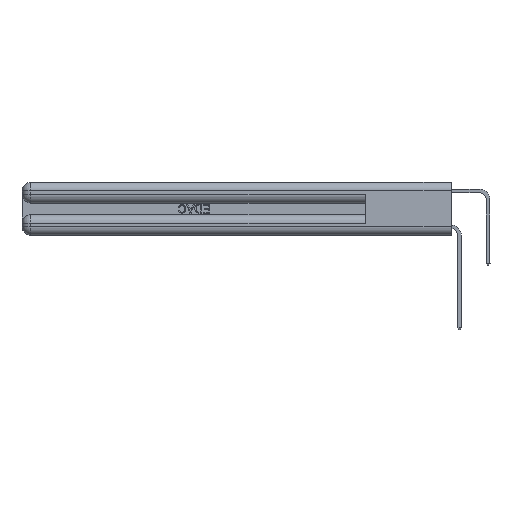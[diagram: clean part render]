
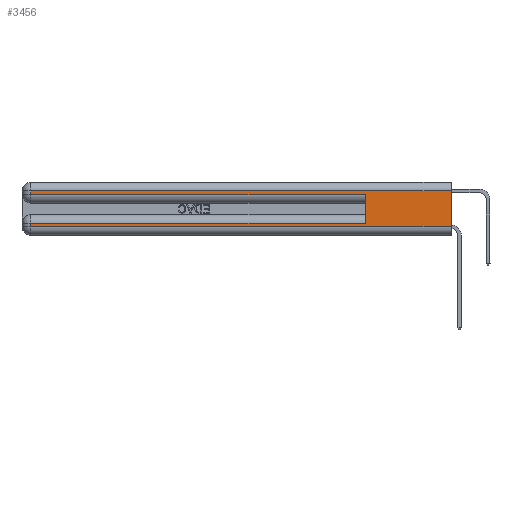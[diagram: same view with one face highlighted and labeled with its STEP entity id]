
A CAD part, left-side view. The second image highlights one B-rep face of the part: STEP entity #3456.
In plain terms, the highlighted planar face has unit normal (-1, 0, 0).
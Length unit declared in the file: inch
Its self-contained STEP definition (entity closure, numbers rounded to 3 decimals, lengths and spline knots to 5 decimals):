
#1261 = ORIENTED_EDGE ( 'NONE', *, *, #28206, .T. ) ;
#2164 = VERTEX_POINT ( 'NONE', #16206 ) ;
#2178 = EDGE_LOOP ( 'NONE', ( #3688, #9739, #6371, #5491, #11661, #1261, #35251, #3676 ) ) ;
#2250 = DIRECTION ( 'NONE',  ( 0., 0., -1. ) ) ;
#2482 = EDGE_CURVE ( 'NONE', #33206, #17365, #23235, .T. ) ;
#2525 = LINE ( 'NONE', #25036, #19591 ) ;
#2604 = FACE_OUTER_BOUND ( 'NONE', #2178, .T. ) ;
#2754 = CARTESIAN_POINT ( 'NONE',  ( 0., 0.6, 0.285 ) ) ;
#3178 = CARTESIAN_POINT ( 'NONE',  ( 0., 2.94, 0.31 ) ) ;
#3456 = ADVANCED_FACE ( 'NONE', ( #2604 ), #27285, .F. ) ;
#3676 = ORIENTED_EDGE ( 'NONE', *, *, #5125, .T. ) ;
#3688 = ORIENTED_EDGE ( 'NONE', *, *, #35032, .F. ) ;
#4379 = DIRECTION ( 'NONE',  ( 0., -1., 0. ) ) ;
#5125 = EDGE_CURVE ( 'NONE', #19645, #2164, #34549, .T. ) ;
#5234 = VECTOR ( 'NONE', #4379, 39.37008 ) ;
#5433 = VERTEX_POINT ( 'NONE', #14145 ) ;
#5491 = ORIENTED_EDGE ( 'NONE', *, *, #6672, .T. ) ;
#5959 = DIRECTION ( 'NONE',  ( 0., 0., -1. ) ) ;
#6371 = ORIENTED_EDGE ( 'NONE', *, *, #25532, .T. ) ;
#6623 = DIRECTION ( 'NONE',  ( 0., 1., 0. ) ) ;
#6672 = EDGE_CURVE ( 'NONE', #34575, #17365, #23557, .T. ) ;
#6862 = CARTESIAN_POINT ( 'NONE',  ( 0., 0., 0.31 ) ) ;
#7670 = VECTOR ( 'NONE', #18965, 39.37008 ) ;
#8605 = VECTOR ( 'NONE', #23261, 39.37008 ) ;
#8687 = LINE ( 'NONE', #27929, #15969 ) ;
#9184 = LINE ( 'NONE', #23133, #9916 ) ;
#9739 = ORIENTED_EDGE ( 'NONE', *, *, #32189, .T. ) ;
#9916 = VECTOR ( 'NONE', #6623, 39.37008 ) ;
#11070 = DIRECTION ( 'NONE',  ( 0., 0., -1. ) ) ;
#11502 = VERTEX_POINT ( 'NONE', #3178 ) ;
#11661 = ORIENTED_EDGE ( 'NONE', *, *, #2482, .F. ) ;
#13624 = VERTEX_POINT ( 'NONE', #6862 ) ;
#14145 = CARTESIAN_POINT ( 'NONE',  ( 0., 2.94, 0.085 ) ) ;
#14431 = EDGE_CURVE ( 'NONE', #5433, #19645, #34548, .T. ) ;
#15689 = CARTESIAN_POINT ( 'NONE',  ( 0., 2.94, 0.06 ) ) ;
#15969 = VECTOR ( 'NONE', #5959, 39.37008 ) ;
#16206 = CARTESIAN_POINT ( 'NONE',  ( 0., 0., 0.06 ) ) ;
#17365 = VERTEX_POINT ( 'NONE', #2754 ) ;
#17774 = CARTESIAN_POINT ( 'NONE',  ( 0., 0.6, 0.145 ) ) ;
#18348 = CARTESIAN_POINT ( 'NONE',  ( 0., 0., 0.06 ) ) ;
#18965 = DIRECTION ( 'NONE',  ( 0., 1., 0. ) ) ;
#19591 = VECTOR ( 'NONE', #11070, 39.37008 ) ;
#19618 = CARTESIAN_POINT ( 'NONE',  ( 0., 2.94, 0.285 ) ) ;
#19645 = VERTEX_POINT ( 'NONE', #15689 ) ;
#20092 = CARTESIAN_POINT ( 'NONE',  ( 0., 0.6, 0.085 ) ) ;
#20697 = CARTESIAN_POINT ( 'NONE',  ( 0., 2.94, 0.37 ) ) ;
#21328 = CARTESIAN_POINT ( 'NONE',  ( 0., 0., 0.31 ) ) ;
#23133 = CARTESIAN_POINT ( 'NONE',  ( 0., 0., 0.085 ) ) ;
#23235 = LINE ( 'NONE', #17774, #31359 ) ;
#23261 = DIRECTION ( 'NONE',  ( 0., 0., -1. ) ) ;
#23380 = CARTESIAN_POINT ( 'NONE',  ( 0., 0., 0.285 ) ) ;
#23557 = LINE ( 'NONE', #23380, #34539 ) ;
#24200 = CARTESIAN_POINT ( 'NONE',  ( 0., 0., 0.37 ) ) ;
#24245 = LINE ( 'NONE', #21328, #7670 ) ;
#25036 = CARTESIAN_POINT ( 'NONE',  ( 0., 0., 0.37 ) ) ;
#25532 = EDGE_CURVE ( 'NONE', #11502, #34575, #8687, .T. ) ;
#27285 = PLANE ( 'NONE',  #29487 ) ;
#27929 = CARTESIAN_POINT ( 'NONE',  ( 0., 2.94, 0.37 ) ) ;
#28206 = EDGE_CURVE ( 'NONE', #33206, #5433, #9184, .T. ) ;
#28872 = DIRECTION ( 'NONE',  ( 0., 0., 1. ) ) ;
#29487 = AXIS2_PLACEMENT_3D ( 'NONE', #24200, #35842, #2250 ) ;
#31359 = VECTOR ( 'NONE', #28872, 39.37008 ) ;
#32189 = EDGE_CURVE ( 'NONE', #13624, #11502, #24245, .T. ) ;
#33206 = VERTEX_POINT ( 'NONE', #20092 ) ;
#34539 = VECTOR ( 'NONE', #35036, 39.37008 ) ;
#34548 = LINE ( 'NONE', #20697, #8605 ) ;
#34549 = LINE ( 'NONE', #18348, #5234 ) ;
#34575 = VERTEX_POINT ( 'NONE', #19618 ) ;
#35032 = EDGE_CURVE ( 'NONE', #13624, #2164, #2525, .T. ) ;
#35036 = DIRECTION ( 'NONE',  ( 0., -1., 0. ) ) ;
#35251 = ORIENTED_EDGE ( 'NONE', *, *, #14431, .T. ) ;
#35842 = DIRECTION ( 'NONE',  ( 1., 0., 0. ) ) ;
